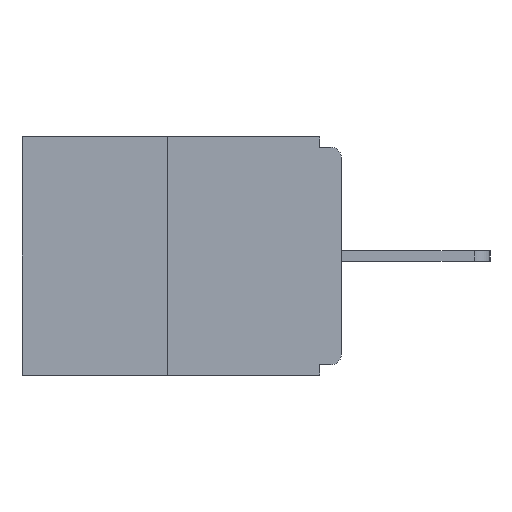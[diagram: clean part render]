
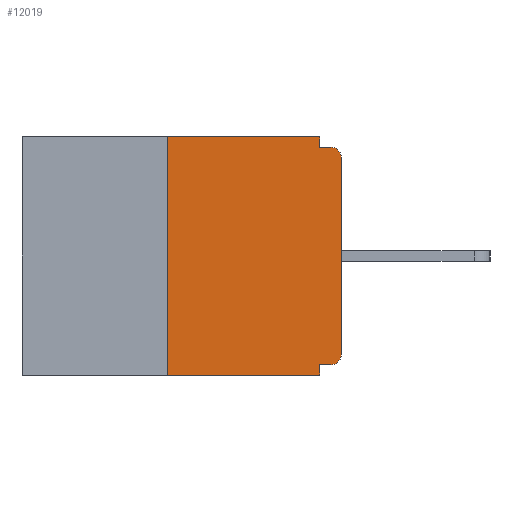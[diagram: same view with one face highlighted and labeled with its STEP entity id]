
A CAD part, left-side view. The second image highlights one B-rep face of the part: STEP entity #12019.
In plain terms, the highlighted planar face has unit normal (-1, 0, 0).
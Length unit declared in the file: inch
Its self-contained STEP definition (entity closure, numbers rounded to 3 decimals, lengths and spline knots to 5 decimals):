
#529 = EDGE_CURVE ( 'NONE', #18067, #23322, #19481, .T. ) ;
#573 = CARTESIAN_POINT ( 'NONE',  ( 0., 0.46, 0. ) ) ;
#694 = DIRECTION ( 'NONE',  ( 0., -1., 0. ) ) ;
#800 = EDGE_CURVE ( 'NONE', #3319, #12697, #20073, .T. ) ;
#1412 = CARTESIAN_POINT ( 'NONE',  ( 0., 0., -0.015 ) ) ;
#1515 = CARTESIAN_POINT ( 'NONE',  ( 0., 0., -0.328 ) ) ;
#2196 = DIRECTION ( 'NONE',  ( 0., 0., -1. ) ) ;
#2202 = AXIS2_PLACEMENT_3D ( 'NONE', #20796, #3608, #9375 ) ;
#2288 = VECTOR ( 'NONE', #16150, 39.37008 ) ;
#2706 = CARTESIAN_POINT ( 'NONE',  ( 0., 0.25, -0.343 ) ) ;
#3319 = VERTEX_POINT ( 'NONE', #10874 ) ;
#3387 = ORIENTED_EDGE ( 'NONE', *, *, #529, .F. ) ;
#3518 = VECTOR ( 'NONE', #2196, 39.37008 ) ;
#3608 = DIRECTION ( 'NONE',  ( -1., 0., 0. ) ) ;
#4796 = EDGE_CURVE ( 'NONE', #10329, #5508, #12338, .T. ) ;
#5011 = ORIENTED_EDGE ( 'NONE', *, *, #22947, .T. ) ;
#5116 = DIRECTION ( 'NONE',  ( 0., 0., -1. ) ) ;
#5217 = ORIENTED_EDGE ( 'NONE', *, *, #16149, .T. ) ;
#5508 = VERTEX_POINT ( 'NONE', #8533 ) ;
#5649 = LINE ( 'NONE', #17324, #15342 ) ;
#5962 = LINE ( 'NONE', #17024, #9189 ) ;
#6551 = ORIENTED_EDGE ( 'NONE', *, *, #21201, .F. ) ;
#6555 = DIRECTION ( 'NONE',  ( -1., 0., 0. ) ) ;
#6612 = VECTOR ( 'NONE', #694, 39.37008 ) ;
#6929 = CIRCLE ( 'NONE', #2202, 0.015 ) ;
#7370 = CARTESIAN_POINT ( 'NONE',  ( 0., 0.031, -0.343 ) ) ;
#7391 = ORIENTED_EDGE ( 'NONE', *, *, #22572, .F. ) ;
#7597 = VECTOR ( 'NONE', #10479, 39.37008 ) ;
#8342 = EDGE_CURVE ( 'NONE', #21636, #12697, #8355, .T. ) ;
#8355 = CIRCLE ( 'NONE', #22090, 0.015 ) ;
#8389 = DIRECTION ( 'NONE',  ( 0., 0., -1. ) ) ;
#8533 = CARTESIAN_POINT ( 'NONE',  ( 0., 0.031, -0.328 ) ) ;
#8675 = CARTESIAN_POINT ( 'NONE',  ( 0., 0.46, 0. ) ) ;
#9189 = VECTOR ( 'NONE', #11127, 39.37008 ) ;
#9349 = EDGE_CURVE ( 'NONE', #15465, #20593, #18960, .T. ) ;
#9375 = DIRECTION ( 'NONE',  ( 0., 0., -1. ) ) ;
#9456 = DIRECTION ( 'NONE',  ( 0., 0., -1. ) ) ;
#10133 = ORIENTED_EDGE ( 'NONE', *, *, #800, .F. ) ;
#10222 = CARTESIAN_POINT ( 'NONE',  ( 0., 0.031, -0.343 ) ) ;
#10329 = VERTEX_POINT ( 'NONE', #12833 ) ;
#10479 = DIRECTION ( 'NONE',  ( 0., -1., 0. ) ) ;
#10874 = CARTESIAN_POINT ( 'NONE',  ( 0., 0.031, -0.015 ) ) ;
#11127 = DIRECTION ( 'NONE',  ( 0., 0., 1. ) ) ;
#12019 = ADVANCED_FACE ( 'NONE', ( #21944 ), #16537, .F. ) ;
#12338 = LINE ( 'NONE', #1515, #2288 ) ;
#12380 = AXIS2_PLACEMENT_3D ( 'NONE', #8675, #12840, #5116 ) ;
#12697 = VERTEX_POINT ( 'NONE', #17921 ) ;
#12833 = CARTESIAN_POINT ( 'NONE',  ( 0., 0.015, -0.328 ) ) ;
#12840 = DIRECTION ( 'NONE',  ( 1., 0., 0. ) ) ;
#13044 = CARTESIAN_POINT ( 'NONE',  ( 0., 0., 0. ) ) ;
#14172 = ORIENTED_EDGE ( 'NONE', *, *, #8342, .T. ) ;
#14473 = EDGE_CURVE ( 'NONE', #15465, #18067, #5962, .T. ) ;
#14847 = LINE ( 'NONE', #13044, #20858 ) ;
#14852 = EDGE_LOOP ( 'NONE', ( #3387, #16969, #17278, #6551, #18011, #5217, #5011, #14172, #10133, #7391 ) ) ;
#14940 = CARTESIAN_POINT ( 'NONE',  ( 0., 0.031, 0. ) ) ;
#15296 = CARTESIAN_POINT ( 'NONE',  ( 0., 0., -0.03 ) ) ;
#15342 = VECTOR ( 'NONE', #9456, 39.37008 ) ;
#15465 = VERTEX_POINT ( 'NONE', #2706 ) ;
#15873 = CARTESIAN_POINT ( 'NONE',  ( 0., 0., -0.313 ) ) ;
#16149 = EDGE_CURVE ( 'NONE', #10329, #22220, #6929, .T. ) ;
#16150 = DIRECTION ( 'NONE',  ( 0., 1., 0. ) ) ;
#16414 = DIRECTION ( 'NONE',  ( 0., -1., 0. ) ) ;
#16537 = PLANE ( 'NONE',  #12380 ) ;
#16969 = ORIENTED_EDGE ( 'NONE', *, *, #14473, .F. ) ;
#17024 = CARTESIAN_POINT ( 'NONE',  ( 0., 0.25, 0. ) ) ;
#17253 = CARTESIAN_POINT ( 'NONE',  ( 0., 0.015, -0.03 ) ) ;
#17278 = ORIENTED_EDGE ( 'NONE', *, *, #9349, .T. ) ;
#17324 = CARTESIAN_POINT ( 'NONE',  ( 0., 0.031, 0. ) ) ;
#17370 = CARTESIAN_POINT ( 'NONE',  ( 0., 0.46, -0.343 ) ) ;
#17921 = CARTESIAN_POINT ( 'NONE',  ( 0., 0.015, -0.015 ) ) ;
#18011 = ORIENTED_EDGE ( 'NONE', *, *, #4796, .F. ) ;
#18067 = VERTEX_POINT ( 'NONE', #23699 ) ;
#18960 = LINE ( 'NONE', #17370, #7597 ) ;
#19481 = LINE ( 'NONE', #573, #6612 ) ;
#20073 = LINE ( 'NONE', #1412, #22668 ) ;
#20593 = VERTEX_POINT ( 'NONE', #10222 ) ;
#20796 = CARTESIAN_POINT ( 'NONE',  ( 0., 0.015, -0.313 ) ) ;
#20858 = VECTOR ( 'NONE', #22342, 39.37008 ) ;
#21201 = EDGE_CURVE ( 'NONE', #5508, #20593, #24207, .T. ) ;
#21636 = VERTEX_POINT ( 'NONE', #15296 ) ;
#21944 = FACE_OUTER_BOUND ( 'NONE', #14852, .T. ) ;
#22090 = AXIS2_PLACEMENT_3D ( 'NONE', #17253, #6555, #8389 ) ;
#22220 = VERTEX_POINT ( 'NONE', #15873 ) ;
#22342 = DIRECTION ( 'NONE',  ( 0., 0., 1. ) ) ;
#22572 = EDGE_CURVE ( 'NONE', #23322, #3319, #5649, .T. ) ;
#22668 = VECTOR ( 'NONE', #16414, 39.37008 ) ;
#22947 = EDGE_CURVE ( 'NONE', #22220, #21636, #14847, .T. ) ;
#23322 = VERTEX_POINT ( 'NONE', #14940 ) ;
#23699 = CARTESIAN_POINT ( 'NONE',  ( 0., 0.25, 0. ) ) ;
#24207 = LINE ( 'NONE', #7370, #3518 ) ;
